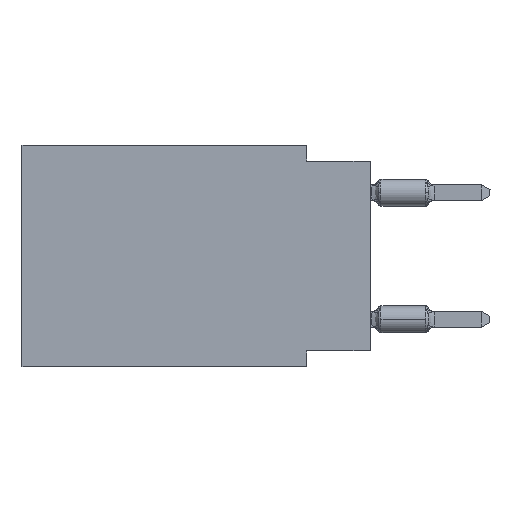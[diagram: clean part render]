
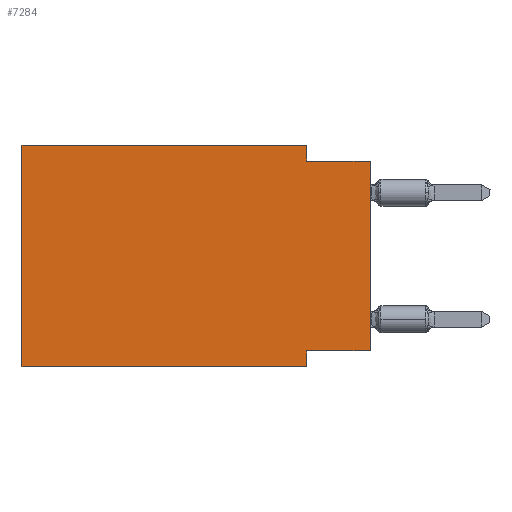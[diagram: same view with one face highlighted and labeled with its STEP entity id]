
A CAD part, left-side view. The second image highlights one B-rep face of the part: STEP entity #7284.
In plain terms, the highlighted planar face has unit normal (-1, 0, 0).
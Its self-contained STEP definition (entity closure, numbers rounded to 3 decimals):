
#65 = CARTESIAN_POINT ( 'NONE',  ( 0., 2.54, 0. ) ) ;
#1129 = CARTESIAN_POINT ( 'NONE',  ( 0., 2.54, -8.255 ) ) ;
#1442 = VERTEX_POINT ( 'NONE', #36277 ) ;
#1752 = CARTESIAN_POINT ( 'NONE',  ( 0., 2.54, -8.89 ) ) ;
#2136 = VECTOR ( 'NONE', #34236, 1000. ) ;
#2322 = LINE ( 'NONE', #7643, #27655 ) ;
#2654 = VERTEX_POINT ( 'NONE', #10616 ) ;
#2660 = VECTOR ( 'NONE', #9998, 1000. ) ;
#2996 = EDGE_CURVE ( 'NONE', #2654, #3577, #9011, .T. ) ;
#3057 = CARTESIAN_POINT ( 'NONE',  ( 0., 13.97, -8.89 ) ) ;
#3291 = VERTEX_POINT ( 'NONE', #3057 ) ;
#3577 = VERTEX_POINT ( 'NONE', #23263 ) ;
#4742 = VECTOR ( 'NONE', #34770, 1000. ) ;
#5057 = CARTESIAN_POINT ( 'NONE',  ( 0., 13.97, 0. ) ) ;
#5810 = CARTESIAN_POINT ( 'NONE',  ( 0., 13.97, 0. ) ) ;
#6111 = VERTEX_POINT ( 'NONE', #65 ) ;
#7284 = ADVANCED_FACE ( 'NONE', ( #32756 ), #29424, .F. ) ;
#7468 = LINE ( 'NONE', #1752, #4742 ) ;
#7643 = CARTESIAN_POINT ( 'NONE',  ( 0., 13.97, -8.89 ) ) ;
#8988 = LINE ( 'NONE', #14695, #21983 ) ;
#9011 = LINE ( 'NONE', #24516, #35001 ) ;
#9575 = DIRECTION ( 'NONE',  ( 0., 0., 1. ) ) ;
#9904 = ORIENTED_EDGE ( 'NONE', *, *, #2996, .T. ) ;
#9998 = DIRECTION ( 'NONE',  ( 0., -1., 0. ) ) ;
#10052 = CARTESIAN_POINT ( 'NONE',  ( 0., 2.54, 0. ) ) ;
#10516 = EDGE_CURVE ( 'NONE', #2654, #35260, #24005, .T. ) ;
#10616 = CARTESIAN_POINT ( 'NONE',  ( 0., 0., -8.255 ) ) ;
#12458 = EDGE_CURVE ( 'NONE', #6111, #14407, #16537, .T. ) ;
#12959 = LINE ( 'NONE', #15695, #2660 ) ;
#13575 = AXIS2_PLACEMENT_3D ( 'NONE', #5810, #23893, #29230 ) ;
#14269 = ORIENTED_EDGE ( 'NONE', *, *, #12458, .F. ) ;
#14407 = VERTEX_POINT ( 'NONE', #28419 ) ;
#14695 = CARTESIAN_POINT ( 'NONE',  ( 0., 13.97, 0. ) ) ;
#15695 = CARTESIAN_POINT ( 'NONE',  ( 0., 0., -0.635 ) ) ;
#16537 = LINE ( 'NONE', #10052, #2136 ) ;
#17052 = DIRECTION ( 'NONE',  ( 0., 0., 1. ) ) ;
#18148 = ORIENTED_EDGE ( 'NONE', *, *, #21197, .F. ) ;
#19119 = EDGE_CURVE ( 'NONE', #3291, #1442, #2322, .T. ) ;
#19352 = EDGE_CURVE ( 'NONE', #25041, #6111, #8988, .T. ) ;
#20194 = EDGE_CURVE ( 'NONE', #3291, #25041, #26683, .T. ) ;
#21197 = EDGE_CURVE ( 'NONE', #14407, #3577, #12959, .T. ) ;
#21731 = ORIENTED_EDGE ( 'NONE', *, *, #28378, .F. ) ;
#21983 = VECTOR ( 'NONE', #29826, 1000. ) ;
#22034 = VECTOR ( 'NONE', #36375, 1000. ) ;
#22120 = ORIENTED_EDGE ( 'NONE', *, *, #20194, .F. ) ;
#23263 = CARTESIAN_POINT ( 'NONE',  ( 0., 0., -0.635 ) ) ;
#23306 = VECTOR ( 'NONE', #17052, 1000. ) ;
#23893 = DIRECTION ( 'NONE',  ( 1., 0., 0. ) ) ;
#24005 = LINE ( 'NONE', #30100, #22034 ) ;
#24231 = EDGE_LOOP ( 'NONE', ( #9904, #18148, #14269, #37787, #22120, #30901, #21731, #32506 ) ) ;
#24516 = CARTESIAN_POINT ( 'NONE',  ( 0., 0., 0. ) ) ;
#25041 = VERTEX_POINT ( 'NONE', #29772 ) ;
#25717 = DIRECTION ( 'NONE',  ( 0., -1., 0. ) ) ;
#26683 = LINE ( 'NONE', #5057, #23306 ) ;
#27655 = VECTOR ( 'NONE', #25717, 1000. ) ;
#28378 = EDGE_CURVE ( 'NONE', #35260, #1442, #7468, .T. ) ;
#28419 = CARTESIAN_POINT ( 'NONE',  ( 0., 2.54, -0.635 ) ) ;
#29230 = DIRECTION ( 'NONE',  ( 0., 0., -1. ) ) ;
#29424 = PLANE ( 'NONE',  #13575 ) ;
#29772 = CARTESIAN_POINT ( 'NONE',  ( 0., 13.97, 0. ) ) ;
#29826 = DIRECTION ( 'NONE',  ( 0., -1., 0. ) ) ;
#30100 = CARTESIAN_POINT ( 'NONE',  ( 0., 0., -8.255 ) ) ;
#30901 = ORIENTED_EDGE ( 'NONE', *, *, #19119, .T. ) ;
#32506 = ORIENTED_EDGE ( 'NONE', *, *, #10516, .F. ) ;
#32756 = FACE_OUTER_BOUND ( 'NONE', #24231, .T. ) ;
#34236 = DIRECTION ( 'NONE',  ( 0., 0., -1. ) ) ;
#34770 = DIRECTION ( 'NONE',  ( 0., 0., -1. ) ) ;
#35001 = VECTOR ( 'NONE', #9575, 1000. ) ;
#35260 = VERTEX_POINT ( 'NONE', #1129 ) ;
#36277 = CARTESIAN_POINT ( 'NONE',  ( 0., 2.54, -8.89 ) ) ;
#36375 = DIRECTION ( 'NONE',  ( 0., 1., 0. ) ) ;
#37787 = ORIENTED_EDGE ( 'NONE', *, *, #19352, .F. ) ;
